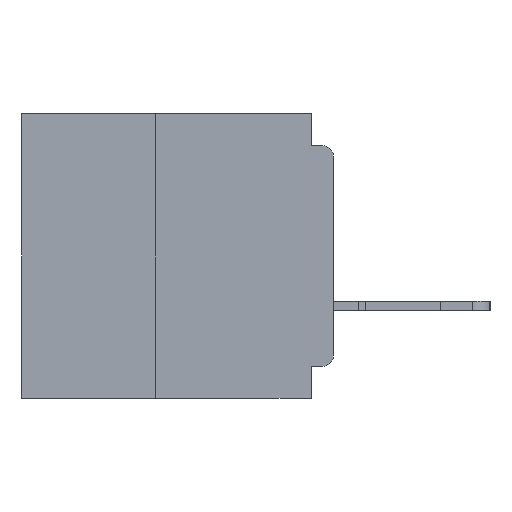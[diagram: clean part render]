
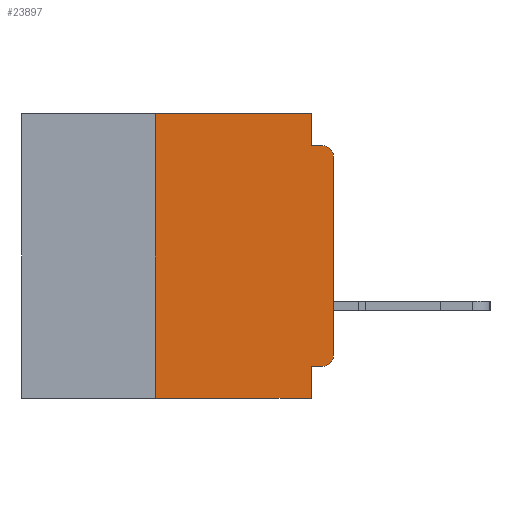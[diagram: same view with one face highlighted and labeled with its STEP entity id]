
A CAD part, left-side view. The second image highlights one B-rep face of the part: STEP entity #23897.
In plain terms, the highlighted planar face has unit normal (-1, 0, 0).
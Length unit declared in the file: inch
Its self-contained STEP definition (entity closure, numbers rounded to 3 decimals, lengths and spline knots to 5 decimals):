
#35 = CARTESIAN_POINT ( 'NONE',  ( 0., 0., -0.355 ) ) ;
#1432 = ORIENTED_EDGE ( 'NONE', *, *, #31106, .F. ) ;
#1597 = EDGE_CURVE ( 'NONE', #60851, #41878, #19802, .T. ) ;
#2251 = EDGE_CURVE ( 'NONE', #41075, #18931, #58824, .T. ) ;
#2324 = DIRECTION ( 'NONE',  ( 0., -1., 0. ) ) ;
#3603 = VECTOR ( 'NONE', #13694, 39.37008 ) ;
#4044 = CARTESIAN_POINT ( 'NONE',  ( 0., 0.031, -0.045 ) ) ;
#4354 = PLANE ( 'NONE',  #40192 ) ;
#4677 = CARTESIAN_POINT ( 'NONE',  ( 0., 0., -0.06 ) ) ;
#6303 = CARTESIAN_POINT ( 'NONE',  ( 0., 0.031, 0. ) ) ;
#6517 = ORIENTED_EDGE ( 'NONE', *, *, #27991, .F. ) ;
#6699 = LINE ( 'NONE', #15416, #18019 ) ;
#6758 = VECTOR ( 'NONE', #2324, 39.37008 ) ;
#7045 = VECTOR ( 'NONE', #20422, 39.37008 ) ;
#8827 = CARTESIAN_POINT ( 'NONE',  ( 0., 0.031, 0. ) ) ;
#9594 = CARTESIAN_POINT ( 'NONE',  ( 0., 0.25, -0.4 ) ) ;
#10067 = LINE ( 'NONE', #58681, #7045 ) ;
#13694 = DIRECTION ( 'NONE',  ( 0., 0., -1. ) ) ;
#14067 = CARTESIAN_POINT ( 'NONE',  ( 0., 0.437, 0. ) ) ;
#14954 = LINE ( 'NONE', #8827, #3603 ) ;
#15416 = CARTESIAN_POINT ( 'NONE',  ( 0., 0.031, -0.4 ) ) ;
#16807 = VECTOR ( 'NONE', #28687, 39.37008 ) ;
#17230 = CARTESIAN_POINT ( 'NONE',  ( 0., 0.015, -0.06 ) ) ;
#17490 = VERTEX_POINT ( 'NONE', #34957 ) ;
#18019 = VECTOR ( 'NONE', #34633, 39.37008 ) ;
#18470 = FACE_OUTER_BOUND ( 'NONE', #40095, .T. ) ;
#18931 = VERTEX_POINT ( 'NONE', #51973 ) ;
#19802 = LINE ( 'NONE', #46334, #45404 ) ;
#20422 = DIRECTION ( 'NONE',  ( 0., 0., 1. ) ) ;
#21507 = CIRCLE ( 'NONE', #55046, 0.015 ) ;
#22141 = DIRECTION ( 'NONE',  ( 0., 0., -1. ) ) ;
#23897 = ADVANCED_FACE ( 'NONE', ( #18470 ), #4354, .F. ) ;
#24218 = CARTESIAN_POINT ( 'NONE',  ( 0., 0.015, -0.355 ) ) ;
#24243 = DIRECTION ( 'NONE',  ( 0., 1., 0. ) ) ;
#25207 = EDGE_CURVE ( 'NONE', #62072, #17490, #36383, .T. ) ;
#26105 = ORIENTED_EDGE ( 'NONE', *, *, #41332, .F. ) ;
#26520 = CARTESIAN_POINT ( 'NONE',  ( 0., 0., -0.045 ) ) ;
#27205 = VERTEX_POINT ( 'NONE', #60555 ) ;
#27991 = EDGE_CURVE ( 'NONE', #41075, #27205, #44321, .T. ) ;
#28687 = DIRECTION ( 'NONE',  ( 0., 0., 1. ) ) ;
#28721 = DIRECTION ( 'NONE',  ( 0., 0., -1. ) ) ;
#29394 = CARTESIAN_POINT ( 'NONE',  ( 0., 0.437, -0.4 ) ) ;
#31106 = EDGE_CURVE ( 'NONE', #62072, #60851, #10067, .T. ) ;
#31598 = EDGE_CURVE ( 'NONE', #18931, #56580, #53688, .T. ) ;
#33841 = VERTEX_POINT ( 'NONE', #45240 ) ;
#33944 = EDGE_CURVE ( 'NONE', #56580, #33841, #21507, .T. ) ;
#34633 = DIRECTION ( 'NONE',  ( 0., 0., -1. ) ) ;
#34957 = CARTESIAN_POINT ( 'NONE',  ( 0., 0.031, -0.4 ) ) ;
#36175 = ORIENTED_EDGE ( 'NONE', *, *, #25207, .T. ) ;
#36383 = LINE ( 'NONE', #29394, #60359 ) ;
#38016 = ORIENTED_EDGE ( 'NONE', *, *, #38174, .F. ) ;
#38174 = EDGE_CURVE ( 'NONE', #41878, #58327, #14954, .T. ) ;
#38196 = AXIS2_PLACEMENT_3D ( 'NONE', #58410, #57982, #57303 ) ;
#40095 = EDGE_LOOP ( 'NONE', ( #61840, #44992, #26105, #38016, #49926, #1432, #36175, #58543, #6517, #52568 ) ) ;
#40192 = AXIS2_PLACEMENT_3D ( 'NONE', #14067, #57398, #28721 ) ;
#41075 = VERTEX_POINT ( 'NONE', #24218 ) ;
#41332 = EDGE_CURVE ( 'NONE', #58327, #33841, #57960, .T. ) ;
#41786 = EDGE_CURVE ( 'NONE', #27205, #17490, #6699, .T. ) ;
#41878 = VERTEX_POINT ( 'NONE', #6303 ) ;
#44321 = LINE ( 'NONE', #35, #55601 ) ;
#44992 = ORIENTED_EDGE ( 'NONE', *, *, #33944, .T. ) ;
#45240 = CARTESIAN_POINT ( 'NONE',  ( 0., 0.015, -0.045 ) ) ;
#45404 = VECTOR ( 'NONE', #46133, 39.37008 ) ;
#46133 = DIRECTION ( 'NONE',  ( 0., -1., 0. ) ) ;
#46334 = CARTESIAN_POINT ( 'NONE',  ( 0., 0.437, 0. ) ) ;
#49926 = ORIENTED_EDGE ( 'NONE', *, *, #1597, .F. ) ;
#50894 = DIRECTION ( 'NONE',  ( -1., 0., 0. ) ) ;
#50955 = CARTESIAN_POINT ( 'NONE',  ( 0., 0.25, 0. ) ) ;
#51973 = CARTESIAN_POINT ( 'NONE',  ( 0., 0., -0.34 ) ) ;
#52568 = ORIENTED_EDGE ( 'NONE', *, *, #2251, .T. ) ;
#52965 = CARTESIAN_POINT ( 'NONE',  ( 0., 0., 0. ) ) ;
#53688 = LINE ( 'NONE', #52965, #16807 ) ;
#55046 = AXIS2_PLACEMENT_3D ( 'NONE', #17230, #50894, #22141 ) ;
#55601 = VECTOR ( 'NONE', #24243, 39.37008 ) ;
#56580 = VERTEX_POINT ( 'NONE', #4677 ) ;
#57303 = DIRECTION ( 'NONE',  ( 0., 0., -1. ) ) ;
#57398 = DIRECTION ( 'NONE',  ( 1., 0., 0. ) ) ;
#57960 = LINE ( 'NONE', #26520, #6758 ) ;
#57982 = DIRECTION ( 'NONE',  ( -1., 0., 0. ) ) ;
#58069 = DIRECTION ( 'NONE',  ( 0., -1., 0. ) ) ;
#58327 = VERTEX_POINT ( 'NONE', #4044 ) ;
#58410 = CARTESIAN_POINT ( 'NONE',  ( 0., 0.015, -0.34 ) ) ;
#58543 = ORIENTED_EDGE ( 'NONE', *, *, #41786, .F. ) ;
#58681 = CARTESIAN_POINT ( 'NONE',  ( 0., 0.25, -0.4 ) ) ;
#58824 = CIRCLE ( 'NONE', #38196, 0.015 ) ;
#60359 = VECTOR ( 'NONE', #58069, 39.37008 ) ;
#60555 = CARTESIAN_POINT ( 'NONE',  ( 0., 0.031, -0.355 ) ) ;
#60851 = VERTEX_POINT ( 'NONE', #50955 ) ;
#61840 = ORIENTED_EDGE ( 'NONE', *, *, #31598, .T. ) ;
#62072 = VERTEX_POINT ( 'NONE', #9594 ) ;
